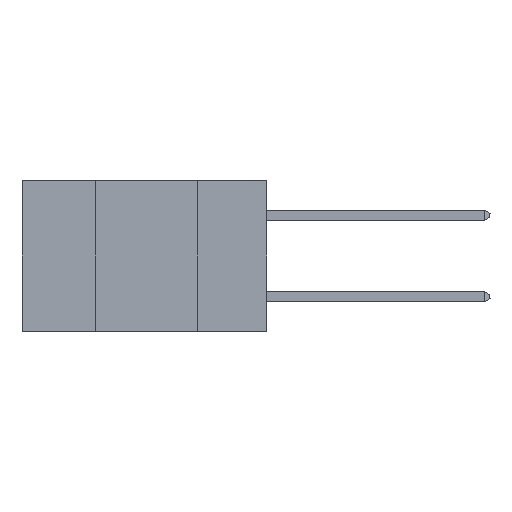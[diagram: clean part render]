
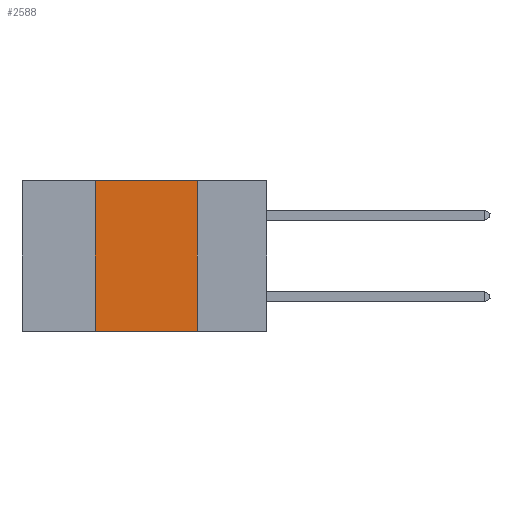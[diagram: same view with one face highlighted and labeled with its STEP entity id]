
A CAD part, left-side view. The second image highlights one B-rep face of the part: STEP entity #2588.
In plain terms, the highlighted planar face has unit normal (-1, 0, 0).
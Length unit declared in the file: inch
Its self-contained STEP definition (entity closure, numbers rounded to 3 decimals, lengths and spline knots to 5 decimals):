
#462 = CARTESIAN_POINT ( 'NONE',  ( 0., 0.6, 0. ) ) ;
#538 = DIRECTION ( 'NONE',  ( 0., 0., -1. ) ) ;
#2588 = ADVANCED_FACE ( 'NONE', ( #20782 ), #22685, .F. ) ;
#3216 = VECTOR ( 'NONE', #4982, 39.37008 ) ;
#3314 = CARTESIAN_POINT ( 'NONE',  ( 0., 0.42, 0. ) ) ;
#3891 = ORIENTED_EDGE ( 'NONE', *, *, #19695, .T. ) ;
#4982 = DIRECTION ( 'NONE',  ( 0., 0., -1. ) ) ;
#5762 = CARTESIAN_POINT ( 'NONE',  ( 0., 0.6, -0.37 ) ) ;
#7081 = CARTESIAN_POINT ( 'NONE',  ( 0., 0.6, 0. ) ) ;
#8755 = CARTESIAN_POINT ( 'NONE',  ( 0., 0.17, 0. ) ) ;
#9116 = EDGE_LOOP ( 'NONE', ( #14580, #16997, #17062, #3891 ) ) ;
#9238 = CARTESIAN_POINT ( 'NONE',  ( 0., 0.17, 0. ) ) ;
#9294 = VERTEX_POINT ( 'NONE', #3314 ) ;
#10089 = VERTEX_POINT ( 'NONE', #9238 ) ;
#10735 = VECTOR ( 'NONE', #21580, 39.37008 ) ;
#11253 = LINE ( 'NONE', #5762, #20973 ) ;
#11777 = DIRECTION ( 'NONE',  ( 1., 0., 0. ) ) ;
#12024 = VECTOR ( 'NONE', #16218, 39.37008 ) ;
#14580 = ORIENTED_EDGE ( 'NONE', *, *, #14779, .F. ) ;
#14779 = EDGE_CURVE ( 'NONE', #10089, #20480, #23412, .T. ) ;
#14840 = EDGE_CURVE ( 'NONE', #9294, #10089, #18059, .T. ) ;
#16185 = LINE ( 'NONE', #19782, #10735 ) ;
#16218 = DIRECTION ( 'NONE',  ( 0., -1., 0. ) ) ;
#16997 = ORIENTED_EDGE ( 'NONE', *, *, #14840, .F. ) ;
#17062 = ORIENTED_EDGE ( 'NONE', *, *, #23744, .F. ) ;
#18059 = LINE ( 'NONE', #7081, #12024 ) ;
#18655 = DIRECTION ( 'NONE',  ( 0., -1., 0. ) ) ;
#19695 = EDGE_CURVE ( 'NONE', #20686, #20480, #11253, .T. ) ;
#19782 = CARTESIAN_POINT ( 'NONE',  ( 0., 0.42, 0. ) ) ;
#20480 = VERTEX_POINT ( 'NONE', #22293 ) ;
#20686 = VERTEX_POINT ( 'NONE', #22823 ) ;
#20782 = FACE_OUTER_BOUND ( 'NONE', #9116, .T. ) ;
#20973 = VECTOR ( 'NONE', #18655, 39.37008 ) ;
#21580 = DIRECTION ( 'NONE',  ( 0., 0., 1. ) ) ;
#22002 = AXIS2_PLACEMENT_3D ( 'NONE', #462, #11777, #538 ) ;
#22293 = CARTESIAN_POINT ( 'NONE',  ( 0., 0.17, -0.37 ) ) ;
#22685 = PLANE ( 'NONE',  #22002 ) ;
#22823 = CARTESIAN_POINT ( 'NONE',  ( 0., 0.42, -0.37 ) ) ;
#23412 = LINE ( 'NONE', #8755, #3216 ) ;
#23744 = EDGE_CURVE ( 'NONE', #20686, #9294, #16185, .T. ) ;
